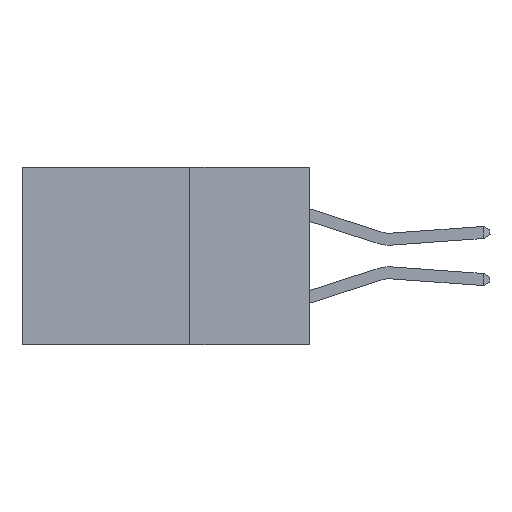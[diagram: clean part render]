
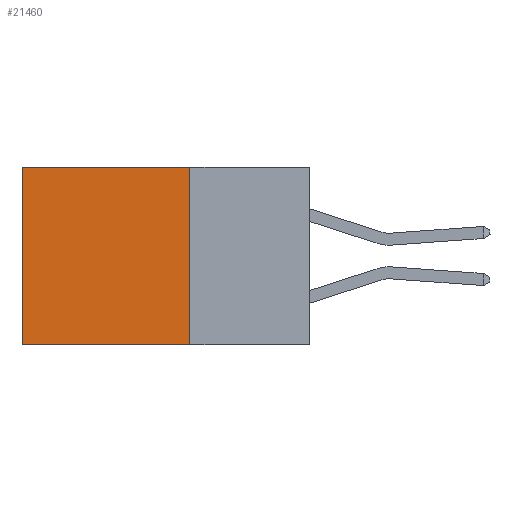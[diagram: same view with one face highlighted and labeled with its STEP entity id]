
A CAD part, left-side view. The second image highlights one B-rep face of the part: STEP entity #21460.
In plain terms, the highlighted planar face has unit normal (-1, 0, 0).
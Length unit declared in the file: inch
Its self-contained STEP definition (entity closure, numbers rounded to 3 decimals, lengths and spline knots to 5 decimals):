
#1006 = LINE ( 'NONE', #21341, #2865 ) ;
#1829 = ORIENTED_EDGE ( 'NONE', *, *, #2272, .F. ) ;
#1839 = EDGE_CURVE ( 'NONE', #5700, #27743, #11559, .T. ) ;
#2272 = EDGE_CURVE ( 'NONE', #24437, #27743, #25207, .T. ) ;
#2465 = CARTESIAN_POINT ( 'NONE',  ( 0.298, 0.6, 0. ) ) ;
#2865 = VECTOR ( 'NONE', #9757, 39.37008 ) ;
#3428 = CARTESIAN_POINT ( 'NONE',  ( 0.298, 0.6, -0.37 ) ) ;
#4475 = CARTESIAN_POINT ( 'NONE',  ( 0.298, 0.25, -0.37 ) ) ;
#5449 = PLANE ( 'NONE',  #10148 ) ;
#5700 = VERTEX_POINT ( 'NONE', #7610 ) ;
#7610 = CARTESIAN_POINT ( 'NONE',  ( 0.298, 0.6, 0. ) ) ;
#9757 = DIRECTION ( 'NONE',  ( 0., 0., -1. ) ) ;
#10029 = CARTESIAN_POINT ( 'NONE',  ( 0.298, 0.25, -0.37 ) ) ;
#10148 = AXIS2_PLACEMENT_3D ( 'NONE', #25211, #11861, #10260 ) ;
#10260 = DIRECTION ( 'NONE',  ( 0., 0., -1. ) ) ;
#11559 = LINE ( 'NONE', #2465, #26741 ) ;
#11861 = DIRECTION ( 'NONE',  ( 1., 0., 0. ) ) ;
#14545 = CARTESIAN_POINT ( 'NONE',  ( 0.298, 0.25, 0. ) ) ;
#15493 = VERTEX_POINT ( 'NONE', #24431 ) ;
#17151 = DIRECTION ( 'NONE',  ( 0., 1., 0. ) ) ;
#17317 = FACE_OUTER_BOUND ( 'NONE', #17880, .T. ) ;
#17880 = EDGE_LOOP ( 'NONE', ( #25474, #1829, #18735, #22313 ) ) ;
#18735 = ORIENTED_EDGE ( 'NONE', *, *, #27250, .F. ) ;
#18744 = DIRECTION ( 'NONE',  ( 0., 0., -1. ) ) ;
#19973 = VECTOR ( 'NONE', #26448, 39.37008 ) ;
#21341 = CARTESIAN_POINT ( 'NONE',  ( 0.298, 0.25, 0. ) ) ;
#21460 = ADVANCED_FACE ( 'NONE', ( #17317 ), #5449, .F. ) ;
#22313 = ORIENTED_EDGE ( 'NONE', *, *, #24933, .T. ) ;
#24431 = CARTESIAN_POINT ( 'NONE',  ( 0.298, 0.25, 0. ) ) ;
#24437 = VERTEX_POINT ( 'NONE', #4475 ) ;
#24933 = EDGE_CURVE ( 'NONE', #15493, #5700, #27811, .T. ) ;
#25207 = LINE ( 'NONE', #10029, #26711 ) ;
#25211 = CARTESIAN_POINT ( 'NONE',  ( 0.298, 0.25, 0. ) ) ;
#25474 = ORIENTED_EDGE ( 'NONE', *, *, #1839, .T. ) ;
#26448 = DIRECTION ( 'NONE',  ( 0., 1., 0. ) ) ;
#26711 = VECTOR ( 'NONE', #17151, 39.37008 ) ;
#26741 = VECTOR ( 'NONE', #18744, 39.37008 ) ;
#27250 = EDGE_CURVE ( 'NONE', #15493, #24437, #1006, .T. ) ;
#27743 = VERTEX_POINT ( 'NONE', #3428 ) ;
#27811 = LINE ( 'NONE', #14545, #19973 ) ;
